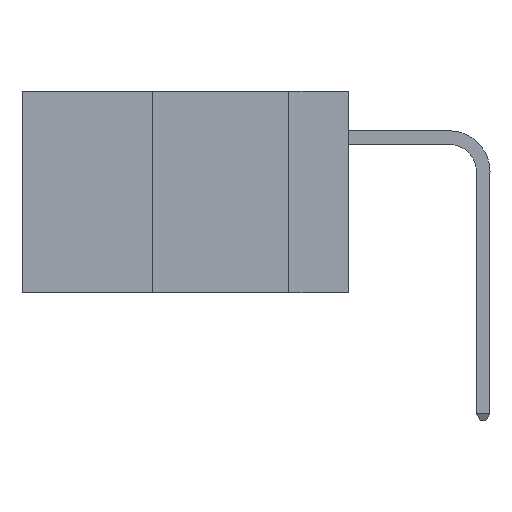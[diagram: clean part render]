
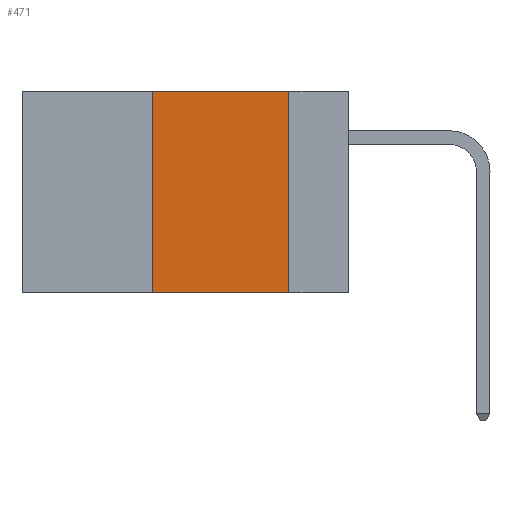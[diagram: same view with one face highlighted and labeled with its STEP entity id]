
A CAD part, left-side view. The second image highlights one B-rep face of the part: STEP entity #471.
In plain terms, the highlighted planar face has unit normal (-1, 0, 0).
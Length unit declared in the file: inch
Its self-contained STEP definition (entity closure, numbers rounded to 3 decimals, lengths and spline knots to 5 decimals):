
#233 = CARTESIAN_POINT ( 'NONE',  ( 0., 0.36, -0.37 ) ) ;
#471 = ADVANCED_FACE ( 'NONE', ( #5937 ), #4196, .F. ) ;
#973 = DIRECTION ( 'NONE',  ( 0., 0., 1. ) ) ;
#1526 = CARTESIAN_POINT ( 'NONE',  ( 0., 0.6, -0.37 ) ) ;
#2867 = EDGE_LOOP ( 'NONE', ( #3895, #5746, #3430, #4286 ) ) ;
#2926 = EDGE_CURVE ( 'NONE', #10468, #3955, #3370, .T. ) ;
#3000 = EDGE_CURVE ( 'NONE', #6526, #5603, #10994, .T. ) ;
#3322 = LINE ( 'NONE', #5662, #7565 ) ;
#3370 = LINE ( 'NONE', #7915, #10432 ) ;
#3430 = ORIENTED_EDGE ( 'NONE', *, *, #3000, .F. ) ;
#3515 = CARTESIAN_POINT ( 'NONE',  ( 0., 0.6, 0. ) ) ;
#3587 = EDGE_CURVE ( 'NONE', #6526, #3955, #4574, .T. ) ;
#3895 = ORIENTED_EDGE ( 'NONE', *, *, #2926, .F. ) ;
#3940 = DIRECTION ( 'NONE',  ( 1., 0., 0. ) ) ;
#3955 = VERTEX_POINT ( 'NONE', #5396 ) ;
#4001 = DIRECTION ( 'NONE',  ( 0., 0., -1. ) ) ;
#4156 = EDGE_CURVE ( 'NONE', #5603, #10468, #3322, .T. ) ;
#4196 = PLANE ( 'NONE',  #4750 ) ;
#4286 = ORIENTED_EDGE ( 'NONE', *, *, #3587, .T. ) ;
#4402 = DIRECTION ( 'NONE',  ( 0., -1., 0. ) ) ;
#4447 = VECTOR ( 'NONE', #973, 39.37008 ) ;
#4574 = LINE ( 'NONE', #1526, #11090 ) ;
#4750 = AXIS2_PLACEMENT_3D ( 'NONE', #3515, #3940, #4001 ) ;
#5396 = CARTESIAN_POINT ( 'NONE',  ( 0., 0.11, -0.37 ) ) ;
#5603 = VERTEX_POINT ( 'NONE', #10877 ) ;
#5662 = CARTESIAN_POINT ( 'NONE',  ( 0., 0.6, 0. ) ) ;
#5746 = ORIENTED_EDGE ( 'NONE', *, *, #4156, .F. ) ;
#5937 = FACE_OUTER_BOUND ( 'NONE', #2867, .T. ) ;
#6526 = VERTEX_POINT ( 'NONE', #233 ) ;
#6570 = CARTESIAN_POINT ( 'NONE',  ( 0., 0.11, 0. ) ) ;
#7565 = VECTOR ( 'NONE', #4402, 39.37008 ) ;
#7629 = DIRECTION ( 'NONE',  ( 0., -1., 0. ) ) ;
#7915 = CARTESIAN_POINT ( 'NONE',  ( 0., 0.11, 0. ) ) ;
#10154 = CARTESIAN_POINT ( 'NONE',  ( 0., 0.36, 0. ) ) ;
#10432 = VECTOR ( 'NONE', #10557, 39.37008 ) ;
#10468 = VERTEX_POINT ( 'NONE', #6570 ) ;
#10557 = DIRECTION ( 'NONE',  ( 0., 0., -1. ) ) ;
#10877 = CARTESIAN_POINT ( 'NONE',  ( 0., 0.36, 0. ) ) ;
#10994 = LINE ( 'NONE', #10154, #4447 ) ;
#11090 = VECTOR ( 'NONE', #7629, 39.37008 ) ;
